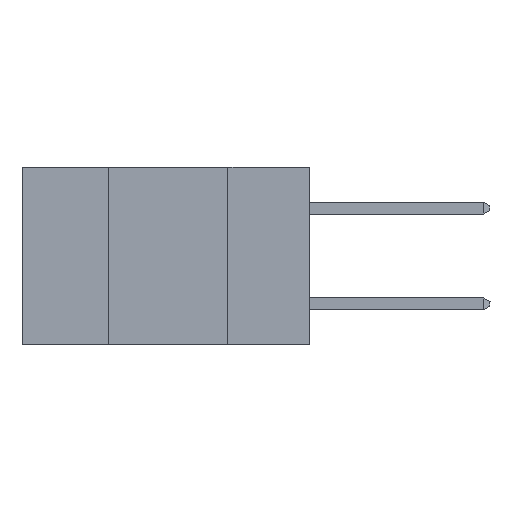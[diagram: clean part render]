
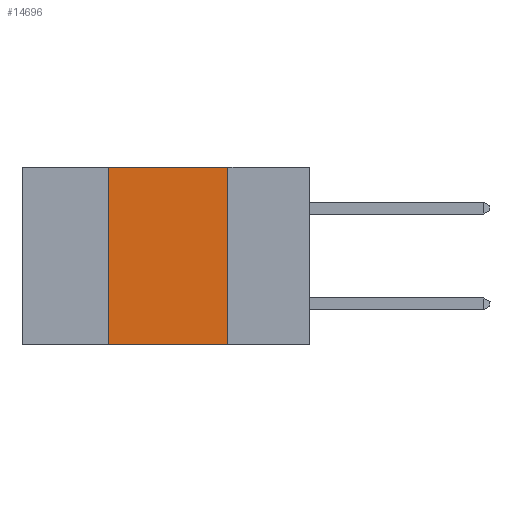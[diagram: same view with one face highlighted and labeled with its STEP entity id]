
A CAD part, left-side view. The second image highlights one B-rep face of the part: STEP entity #14696.
In plain terms, the highlighted planar face has unit normal (-1, 0, 0).
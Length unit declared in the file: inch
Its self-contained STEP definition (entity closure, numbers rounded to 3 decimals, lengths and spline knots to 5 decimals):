
#579 = DIRECTION ( 'NONE',  ( 1., 0., 0. ) ) ;
#751 = EDGE_CURVE ( 'NONE', #13287, #19707, #23799, .T. ) ;
#2440 = AXIS2_PLACEMENT_3D ( 'NONE', #15871, #579, #22089 ) ;
#2818 = VECTOR ( 'NONE', #24067, 39.37008 ) ;
#3084 = CARTESIAN_POINT ( 'NONE',  ( 0., 0.42, -0.37 ) ) ;
#4303 = DIRECTION ( 'NONE',  ( 0., -1., 0. ) ) ;
#8767 = FACE_OUTER_BOUND ( 'NONE', #10899, .T. ) ;
#10621 = ORIENTED_EDGE ( 'NONE', *, *, #21278, .F. ) ;
#10899 = EDGE_LOOP ( 'NONE', ( #24898, #10621, #24432, #17173 ) ) ;
#11489 = VERTEX_POINT ( 'NONE', #20019 ) ;
#12310 = VECTOR ( 'NONE', #22008, 39.37008 ) ;
#12425 = CARTESIAN_POINT ( 'NONE',  ( 0., 0.42, 0. ) ) ;
#13287 = VERTEX_POINT ( 'NONE', #3084 ) ;
#14363 = CARTESIAN_POINT ( 'NONE',  ( 0., 0.42, 0. ) ) ;
#14696 = ADVANCED_FACE ( 'NONE', ( #8767 ), #20398, .F. ) ;
#15871 = CARTESIAN_POINT ( 'NONE',  ( 0., 0.6, 0. ) ) ;
#16242 = LINE ( 'NONE', #12425, #26685 ) ;
#17173 = ORIENTED_EDGE ( 'NONE', *, *, #751, .T. ) ;
#18570 = EDGE_CURVE ( 'NONE', #13287, #27743, #16242, .T. ) ;
#19627 = CARTESIAN_POINT ( 'NONE',  ( 0., 0.6, 0. ) ) ;
#19707 = VERTEX_POINT ( 'NONE', #27128 ) ;
#20019 = CARTESIAN_POINT ( 'NONE',  ( 0., 0.17, 0. ) ) ;
#20379 = LINE ( 'NONE', #21724, #2818 ) ;
#20398 = PLANE ( 'NONE',  #2440 ) ;
#21278 = EDGE_CURVE ( 'NONE', #27743, #11489, #27854, .T. ) ;
#21724 = CARTESIAN_POINT ( 'NONE',  ( 0., 0.17, 0. ) ) ;
#22008 = DIRECTION ( 'NONE',  ( 0., -1., 0. ) ) ;
#22089 = DIRECTION ( 'NONE',  ( 0., 0., -1. ) ) ;
#23799 = LINE ( 'NONE', #24066, #12310 ) ;
#24066 = CARTESIAN_POINT ( 'NONE',  ( 0., 0.6, -0.37 ) ) ;
#24067 = DIRECTION ( 'NONE',  ( 0., 0., -1. ) ) ;
#24432 = ORIENTED_EDGE ( 'NONE', *, *, #18570, .F. ) ;
#24898 = ORIENTED_EDGE ( 'NONE', *, *, #25142, .F. ) ;
#25142 = EDGE_CURVE ( 'NONE', #11489, #19707, #20379, .T. ) ;
#25253 = DIRECTION ( 'NONE',  ( 0., 0., 1. ) ) ;
#26503 = VECTOR ( 'NONE', #4303, 39.37008 ) ;
#26685 = VECTOR ( 'NONE', #25253, 39.37008 ) ;
#27128 = CARTESIAN_POINT ( 'NONE',  ( 0., 0.17, -0.37 ) ) ;
#27743 = VERTEX_POINT ( 'NONE', #14363 ) ;
#27854 = LINE ( 'NONE', #19627, #26503 ) ;
